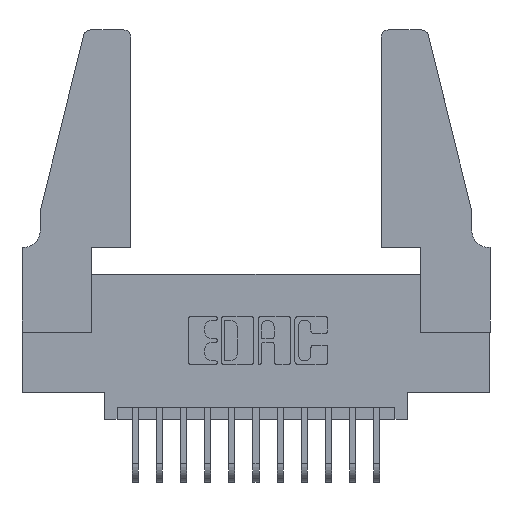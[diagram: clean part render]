
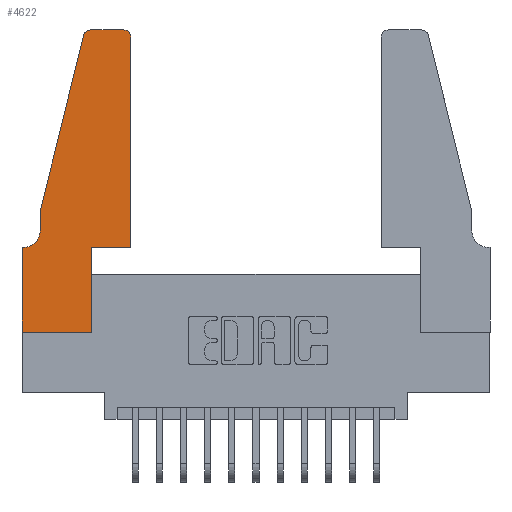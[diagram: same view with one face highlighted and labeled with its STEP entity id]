
A CAD part, top view. The second image highlights one B-rep face of the part: STEP entity #4622.
In plain terms, the highlighted planar face has unit normal (0, 0, 1).
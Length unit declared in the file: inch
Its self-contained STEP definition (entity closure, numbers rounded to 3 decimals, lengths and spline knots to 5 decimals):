
#4 = LINE ( 'NONE', #5521, #16398 ) ;
#172 = ORIENTED_EDGE ( 'NONE', *, *, #2939, .T. ) ;
#372 = VECTOR ( 'NONE', #9009, 39.37008 ) ;
#401 = CARTESIAN_POINT ( 'NONE',  ( 0.2865, 0.35, 0.37 ) ) ;
#430 = DIRECTION ( 'NONE',  ( 0., -1., 0. ) ) ;
#685 = VERTEX_POINT ( 'NONE', #5749 ) ;
#936 = LINE ( 'NONE', #12489, #5112 ) ;
#948 = VECTOR ( 'NONE', #2932, 39.37008 ) ;
#1691 = ORIENTED_EDGE ( 'NONE', *, *, #6785, .T. ) ;
#2084 = DIRECTION ( 'NONE',  ( 0., 0., 1. ) ) ;
#2447 = VERTEX_POINT ( 'NONE', #8606 ) ;
#2932 = DIRECTION ( 'NONE',  ( -1., 0., 0. ) ) ;
#2936 = CARTESIAN_POINT ( 'NONE',  ( 0.284, 1.25, 0.37 ) ) ;
#2939 = EDGE_CURVE ( 'NONE', #15070, #5568, #15890, .T. ) ;
#2949 = PLANE ( 'NONE',  #9130 ) ;
#3202 = VERTEX_POINT ( 'NONE', #6483 ) ;
#3315 = EDGE_CURVE ( 'NONE', #5568, #2447, #13658, .T. ) ;
#3438 = VERTEX_POINT ( 'NONE', #10880 ) ;
#3619 = FACE_OUTER_BOUND ( 'NONE', #14574, .T. ) ;
#3765 = LINE ( 'NONE', #12864, #372 ) ;
#3815 = VECTOR ( 'NONE', #15153, 39.37008 ) ;
#3951 = EDGE_CURVE ( 'NONE', #4850, #7984, #4648, .T. ) ;
#4007 = LINE ( 'NONE', #9475, #11412 ) ;
#4204 = CARTESIAN_POINT ( 'NONE',  ( 0., 0., 0.37 ) ) ;
#4312 = CARTESIAN_POINT ( 'NONE',  ( 0.0055, 0.35, 0.37 ) ) ;
#4609 = EDGE_CURVE ( 'NONE', #13901, #7446, #4007, .T. ) ;
#4622 = ADVANCED_FACE ( 'NONE', ( #3619 ), #2949, .T. ) ;
#4646 = DIRECTION ( 'NONE',  ( 1., 0., 0. ) ) ;
#4648 = LINE ( 'NONE', #4204, #10806 ) ;
#4850 = VERTEX_POINT ( 'NONE', #6018 ) ;
#4940 = DIRECTION ( 'NONE',  ( 0., 0., 1. ) ) ;
#5112 = VECTOR ( 'NONE', #4646, 39.37008 ) ;
#5117 = ORIENTED_EDGE ( 'NONE', *, *, #3951, .T. ) ;
#5209 = ORIENTED_EDGE ( 'NONE', *, *, #10727, .T. ) ;
#5521 = CARTESIAN_POINT ( 'NONE',  ( 0.0755, 0.5, 0.37 ) ) ;
#5548 = CARTESIAN_POINT ( 'NONE',  ( 0., 0.35, 0.37 ) ) ;
#5568 = VERTEX_POINT ( 'NONE', #13931 ) ;
#5702 = EDGE_CURVE ( 'NONE', #2447, #3438, #4, .T. ) ;
#5749 = CARTESIAN_POINT ( 'NONE',  ( 0.4205, 1.25, 0.37 ) ) ;
#6018 = CARTESIAN_POINT ( 'NONE',  ( 0., 0.35, 0.37 ) ) ;
#6137 = EDGE_CURVE ( 'NONE', #12965, #13901, #3765, .T. ) ;
#6315 = CARTESIAN_POINT ( 'NONE',  ( 0.2865, 0.35, 0.37 ) ) ;
#6483 = CARTESIAN_POINT ( 'NONE',  ( 0.2865, 0., 0.37 ) ) ;
#6613 = ORIENTED_EDGE ( 'NONE', *, *, #6137, .T. ) ;
#6766 = CARTESIAN_POINT ( 'NONE',  ( 0.0055, 0.42, 0.37 ) ) ;
#6785 = EDGE_CURVE ( 'NONE', #7446, #685, #11712, .T. ) ;
#6814 = CARTESIAN_POINT ( 'NONE',  ( 0.2605, 1.25, 0.37 ) ) ;
#6893 = DIRECTION ( 'NONE',  ( 1., 0., 0. ) ) ;
#7446 = VERTEX_POINT ( 'NONE', #15529 ) ;
#7523 = CIRCLE ( 'NONE', #14917, 0.07 ) ;
#7984 = VERTEX_POINT ( 'NONE', #12758 ) ;
#8104 = DIRECTION ( 'NONE',  ( -1., 0., 0. ) ) ;
#8340 = ORIENTED_EDGE ( 'NONE', *, *, #5702, .T. ) ;
#8606 = CARTESIAN_POINT ( 'NONE',  ( 0.0755, 0.5, 0.37 ) ) ;
#8707 = CARTESIAN_POINT ( 'NONE',  ( 0.0755, 0.35, 0.37 ) ) ;
#9009 = DIRECTION ( 'NONE',  ( 1., 0., 0. ) ) ;
#9130 = AXIS2_PLACEMENT_3D ( 'NONE', #5548, #14686, #6893 ) ;
#9407 = ORIENTED_EDGE ( 'NONE', *, *, #10460, .T. ) ;
#9475 = CARTESIAN_POINT ( 'NONE',  ( 0.4505, 0.35, 0.37 ) ) ;
#9802 = ORIENTED_EDGE ( 'NONE', *, *, #14645, .T. ) ;
#9866 = CARTESIAN_POINT ( 'NONE',  ( 0.284, 1.22, 0.37 ) ) ;
#10460 = EDGE_CURVE ( 'NONE', #15773, #4850, #15442, .T. ) ;
#10727 = EDGE_CURVE ( 'NONE', #3438, #15773, #7523, .T. ) ;
#10788 = DIRECTION ( 'NONE',  ( 0., 1., 0. ) ) ;
#10806 = VECTOR ( 'NONE', #430, 39.37008 ) ;
#10880 = CARTESIAN_POINT ( 'NONE',  ( 0.0755, 0.42, 0.37 ) ) ;
#11143 = ORIENTED_EDGE ( 'NONE', *, *, #13244, .T. ) ;
#11193 = DIRECTION ( 'NONE',  ( 1., 0., 0. ) ) ;
#11412 = VECTOR ( 'NONE', #10788, 39.37008 ) ;
#11512 = VECTOR ( 'NONE', #16721, 39.37008 ) ;
#11712 = CIRCLE ( 'NONE', #16494, 0.03 ) ;
#12060 = DIRECTION ( 'NONE',  ( 0., -1., 0. ) ) ;
#12296 = LINE ( 'NONE', #6315, #11512 ) ;
#12489 = CARTESIAN_POINT ( 'NONE',  ( 0., 0., 0.37 ) ) ;
#12758 = CARTESIAN_POINT ( 'NONE',  ( 0., 0., 0.37 ) ) ;
#12791 = CARTESIAN_POINT ( 'NONE',  ( 0.4205, 1.22, 0.37 ) ) ;
#12806 = AXIS2_PLACEMENT_3D ( 'NONE', #9866, #2084, #11193 ) ;
#12864 = CARTESIAN_POINT ( 'NONE',  ( 0.4505, 0.35, 0.37 ) ) ;
#12965 = VERTEX_POINT ( 'NONE', #401 ) ;
#13152 = CARTESIAN_POINT ( 'NONE',  ( 0.0755, 0.5, 0.37 ) ) ;
#13244 = EDGE_CURVE ( 'NONE', #3202, #12965, #12296, .T. ) ;
#13475 = EDGE_CURVE ( 'NONE', #685, #15070, #14719, .T. ) ;
#13658 = LINE ( 'NONE', #13152, #16698 ) ;
#13901 = VERTEX_POINT ( 'NONE', #14228 ) ;
#13919 = ORIENTED_EDGE ( 'NONE', *, *, #4609, .T. ) ;
#13931 = CARTESIAN_POINT ( 'NONE',  ( 0.25487, 1.22718, 0.37 ) ) ;
#14086 = DIRECTION ( 'NONE',  ( 1., 0., 0. ) ) ;
#14228 = CARTESIAN_POINT ( 'NONE',  ( 0.4505, 0.35, 0.37 ) ) ;
#14574 = EDGE_LOOP ( 'NONE', ( #16613, #172, #14810, #8340, #5209, #9407, #5117, #9802, #11143, #6613, #13919, #1691 ) ) ;
#14645 = EDGE_CURVE ( 'NONE', #7984, #3202, #936, .T. ) ;
#14686 = DIRECTION ( 'NONE',  ( 0., 0., 1. ) ) ;
#14719 = LINE ( 'NONE', #6814, #948 ) ;
#14810 = ORIENTED_EDGE ( 'NONE', *, *, #3315, .T. ) ;
#14917 = AXIS2_PLACEMENT_3D ( 'NONE', #6766, #15859, #8104 ) ;
#15070 = VERTEX_POINT ( 'NONE', #2936 ) ;
#15153 = DIRECTION ( 'NONE',  ( -1., 0., 0. ) ) ;
#15442 = LINE ( 'NONE', #8707, #3815 ) ;
#15529 = CARTESIAN_POINT ( 'NONE',  ( 0.4505, 1.22, 0.37 ) ) ;
#15773 = VERTEX_POINT ( 'NONE', #4312 ) ;
#15788 = DIRECTION ( 'NONE',  ( -0.239, -0.971, 0. ) ) ;
#15859 = DIRECTION ( 'NONE',  ( 0., 0., -1. ) ) ;
#15890 = CIRCLE ( 'NONE', #12806, 0.03 ) ;
#16398 = VECTOR ( 'NONE', #12060, 39.37008 ) ;
#16494 = AXIS2_PLACEMENT_3D ( 'NONE', #12791, #4940, #14086 ) ;
#16613 = ORIENTED_EDGE ( 'NONE', *, *, #13475, .T. ) ;
#16698 = VECTOR ( 'NONE', #15788, 39.37008 ) ;
#16721 = DIRECTION ( 'NONE',  ( 0., 1., 0. ) ) ;
